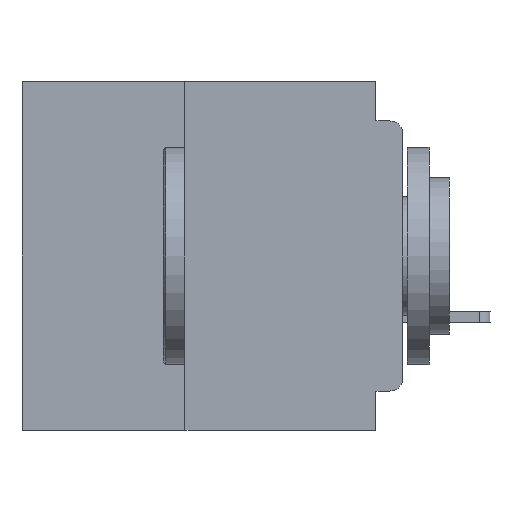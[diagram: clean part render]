
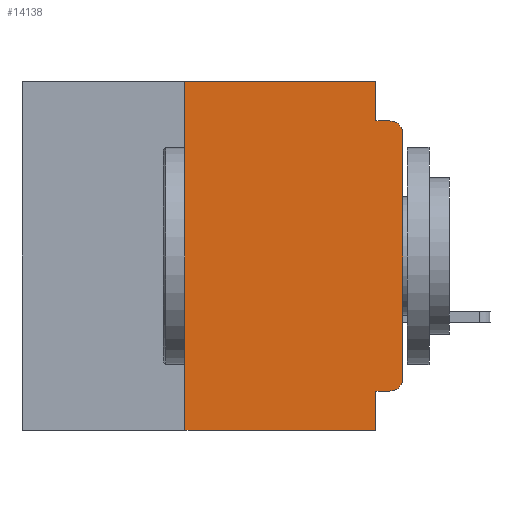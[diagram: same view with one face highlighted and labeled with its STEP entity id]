
A CAD part, left-side view. The second image highlights one B-rep face of the part: STEP entity #14138.
In plain terms, the highlighted planar face has unit normal (-1, 0, 0).
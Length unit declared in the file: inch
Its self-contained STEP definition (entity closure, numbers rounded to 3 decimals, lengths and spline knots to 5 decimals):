
#192 = CARTESIAN_POINT ( 'NONE',  ( 0., 0., 0. ) ) ;
#1004 = FACE_OUTER_BOUND ( 'NONE', #30032, .T. ) ;
#1691 = VECTOR ( 'NONE', #38523, 39.37008 ) ;
#2513 = DIRECTION ( 'NONE',  ( 0., 1., 0. ) ) ;
#4227 = ORIENTED_EDGE ( 'NONE', *, *, #23995, .T. ) ;
#4646 = LINE ( 'NONE', #53663, #51585 ) ;
#5295 = CIRCLE ( 'NONE', #16098, 0.015 ) ;
#7564 = DIRECTION ( 'NONE',  ( -1., 0., 0. ) ) ;
#8075 = VECTOR ( 'NONE', #17092, 39.37008 ) ;
#8657 = CARTESIAN_POINT ( 'NONE',  ( 0., 0.25, 0. ) ) ;
#8853 = VERTEX_POINT ( 'NONE', #17039 ) ;
#9306 = CARTESIAN_POINT ( 'NONE',  ( 0., 0.031, -0.355 ) ) ;
#9538 = ORIENTED_EDGE ( 'NONE', *, *, #17904, .T. ) ;
#10443 = VECTOR ( 'NONE', #46663, 39.37008 ) ;
#10556 = DIRECTION ( 'NONE',  ( 0., 0., 1. ) ) ;
#11803 = VERTEX_POINT ( 'NONE', #14814 ) ;
#12275 = VERTEX_POINT ( 'NONE', #13725 ) ;
#13025 = DIRECTION ( 'NONE',  ( 0., -1., 0. ) ) ;
#13725 = CARTESIAN_POINT ( 'NONE',  ( 0., 0.015, -0.355 ) ) ;
#13821 = EDGE_CURVE ( 'NONE', #38442, #35179, #4646, .T. ) ;
#14089 = DIRECTION ( 'NONE',  ( 0., 0., 1. ) ) ;
#14138 = ADVANCED_FACE ( 'NONE', ( #1004 ), #55773, .F. ) ;
#14669 = CARTESIAN_POINT ( 'NONE',  ( 0., 0.015, -0.06 ) ) ;
#14814 = CARTESIAN_POINT ( 'NONE',  ( 0., 0.031, 0. ) ) ;
#14946 = CARTESIAN_POINT ( 'NONE',  ( 0., 0.031, 0. ) ) ;
#14969 = CARTESIAN_POINT ( 'NONE',  ( 0., 0.437, 0. ) ) ;
#15225 = CARTESIAN_POINT ( 'NONE',  ( 0., 0.25, -0.4 ) ) ;
#15227 = ORIENTED_EDGE ( 'NONE', *, *, #18781, .F. ) ;
#15249 = DIRECTION ( 'NONE',  ( 1., 0., 0. ) ) ;
#16098 = AXIS2_PLACEMENT_3D ( 'NONE', #14669, #46393, #19257 ) ;
#17039 = CARTESIAN_POINT ( 'NONE',  ( 0., 0.031, -0.045 ) ) ;
#17092 = DIRECTION ( 'NONE',  ( 0., 0., -1. ) ) ;
#17904 = EDGE_CURVE ( 'NONE', #47773, #36305, #31211, .T. ) ;
#18781 = EDGE_CURVE ( 'NONE', #12275, #31347, #28243, .T. ) ;
#19139 = ORIENTED_EDGE ( 'NONE', *, *, #44866, .F. ) ;
#19257 = DIRECTION ( 'NONE',  ( 0., 0., -1. ) ) ;
#20316 = LINE ( 'NONE', #35228, #8075 ) ;
#21963 = VERTEX_POINT ( 'NONE', #55005 ) ;
#23995 = EDGE_CURVE ( 'NONE', #12275, #47773, #31542, .T. ) ;
#24837 = CARTESIAN_POINT ( 'NONE',  ( 0., 0., -0.045 ) ) ;
#27076 = CARTESIAN_POINT ( 'NONE',  ( 0., 0.25, -0.4 ) ) ;
#28243 = LINE ( 'NONE', #56929, #40276 ) ;
#29782 = VECTOR ( 'NONE', #14089, 39.37008 ) ;
#29862 = EDGE_CURVE ( 'NONE', #49307, #11803, #49208, .T. ) ;
#30032 = EDGE_LOOP ( 'NONE', ( #9538, #37207, #48470, #33124, #37349, #19139, #40687, #55180, #15227, #4227 ) ) ;
#30548 = LINE ( 'NONE', #15225, #53111 ) ;
#31211 = LINE ( 'NONE', #192, #29782 ) ;
#31347 = VERTEX_POINT ( 'NONE', #9306 ) ;
#31542 = CIRCLE ( 'NONE', #49889, 0.015 ) ;
#33124 = ORIENTED_EDGE ( 'NONE', *, *, #49975, .F. ) ;
#33386 = CARTESIAN_POINT ( 'NONE',  ( 0., 0.437, 0. ) ) ;
#34514 = CARTESIAN_POINT ( 'NONE',  ( 0., 0., -0.06 ) ) ;
#34966 = CARTESIAN_POINT ( 'NONE',  ( 0., 0.015, -0.34 ) ) ;
#35179 = VERTEX_POINT ( 'NONE', #35537 ) ;
#35228 = CARTESIAN_POINT ( 'NONE',  ( 0., 0.031, -0.4 ) ) ;
#35537 = CARTESIAN_POINT ( 'NONE',  ( 0., 0.031, -0.4 ) ) ;
#36280 = AXIS2_PLACEMENT_3D ( 'NONE', #33386, #15249, #46968 ) ;
#36305 = VERTEX_POINT ( 'NONE', #34514 ) ;
#37207 = ORIENTED_EDGE ( 'NONE', *, *, #53151, .T. ) ;
#37258 = VECTOR ( 'NONE', #55699, 39.37008 ) ;
#37349 = ORIENTED_EDGE ( 'NONE', *, *, #29862, .F. ) ;
#38442 = VERTEX_POINT ( 'NONE', #27076 ) ;
#38523 = DIRECTION ( 'NONE',  ( 0., -1., 0. ) ) ;
#39479 = DIRECTION ( 'NONE',  ( 0., 0., -1. ) ) ;
#40276 = VECTOR ( 'NONE', #2513, 39.37008 ) ;
#40687 = ORIENTED_EDGE ( 'NONE', *, *, #13821, .T. ) ;
#44866 = EDGE_CURVE ( 'NONE', #38442, #49307, #30548, .T. ) ;
#45287 = LINE ( 'NONE', #14946, #10443 ) ;
#46167 = EDGE_CURVE ( 'NONE', #8853, #21963, #51529, .T. ) ;
#46393 = DIRECTION ( 'NONE',  ( -1., 0., 0. ) ) ;
#46663 = DIRECTION ( 'NONE',  ( 0., 0., -1. ) ) ;
#46968 = DIRECTION ( 'NONE',  ( 0., 0., -1. ) ) ;
#47773 = VERTEX_POINT ( 'NONE', #55622 ) ;
#48470 = ORIENTED_EDGE ( 'NONE', *, *, #46167, .F. ) ;
#49208 = LINE ( 'NONE', #14969, #37258 ) ;
#49307 = VERTEX_POINT ( 'NONE', #8657 ) ;
#49889 = AXIS2_PLACEMENT_3D ( 'NONE', #34966, #7564, #39479 ) ;
#49975 = EDGE_CURVE ( 'NONE', #11803, #8853, #45287, .T. ) ;
#51529 = LINE ( 'NONE', #24837, #1691 ) ;
#51585 = VECTOR ( 'NONE', #13025, 39.37008 ) ;
#52181 = EDGE_CURVE ( 'NONE', #31347, #35179, #20316, .T. ) ;
#53111 = VECTOR ( 'NONE', #10556, 39.37008 ) ;
#53151 = EDGE_CURVE ( 'NONE', #36305, #21963, #5295, .T. ) ;
#53663 = CARTESIAN_POINT ( 'NONE',  ( 0., 0.437, -0.4 ) ) ;
#55005 = CARTESIAN_POINT ( 'NONE',  ( 0., 0.015, -0.045 ) ) ;
#55180 = ORIENTED_EDGE ( 'NONE', *, *, #52181, .F. ) ;
#55622 = CARTESIAN_POINT ( 'NONE',  ( 0., 0., -0.34 ) ) ;
#55699 = DIRECTION ( 'NONE',  ( 0., -1., 0. ) ) ;
#55773 = PLANE ( 'NONE',  #36280 ) ;
#56929 = CARTESIAN_POINT ( 'NONE',  ( 0., 0., -0.355 ) ) ;
